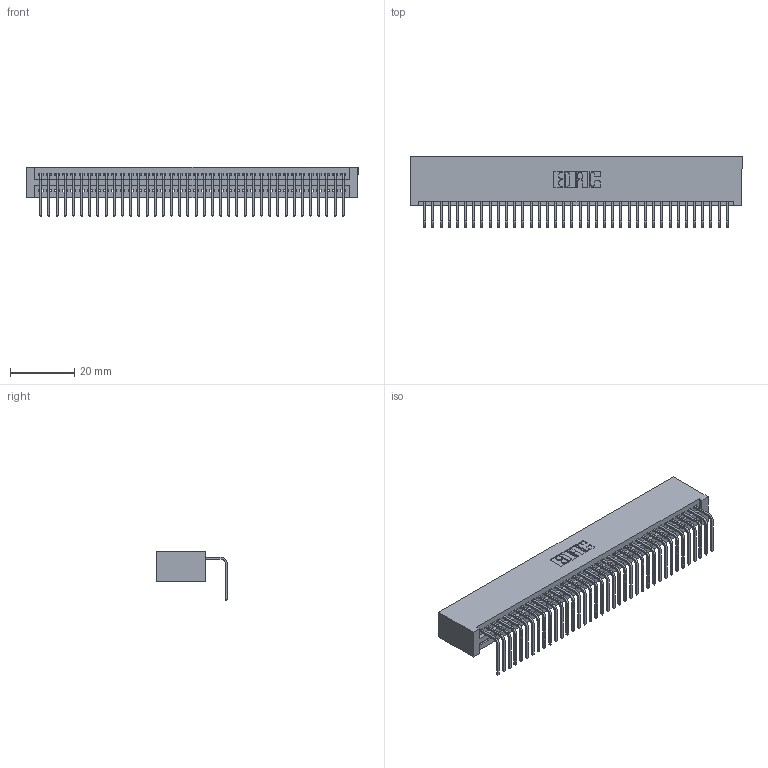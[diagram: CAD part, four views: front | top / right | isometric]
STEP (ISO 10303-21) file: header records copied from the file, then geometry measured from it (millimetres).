
FILE_DESCRIPTION (( 'STEP AP203' ), '1' );
FILE_NAME ('395-038-558-101.STEP', '2019-10-11T11:13:30', ( '' ), ( '' ), 'SwSTEP 2.0', 'SolidWorks 2016', '' );
FILE_SCHEMA (( 'CONFIG_CONTROL_DESIGN' ));
Length unit declared in the file: inch
Products named in the file (3): 345 Part_No Mounting Lugs; 345-292-001_558 Tail - 2; 395-038-558-101
Assembly tree (39 placements, depth 2):
  395-038-558-101
    345 Part_No Mounting Lugs
    345-292-001_558 Tail - 2  x38
Bounding box: 103.12 x 21.83 x 15.37 mm (x, y, z)
Volume: 10473 mm3; surface area: 14797.4 mm2
Topology: 39 solids, 39 shells, 2398 faces, 7233 edges, 4770 vertices
Faces by surface type: plane 1672, cylinder 726
Entity records: 28945 total; most frequent: CARTESIAN_POINT 5022, ORIENTED_EDGE 4994, DIRECTION 4385, EDGE_CURVE 2497, VECTOR 2221, LINE 2221, VERTEX_POINT 1662, AXIS2_PLACEMENT_3D 1082
